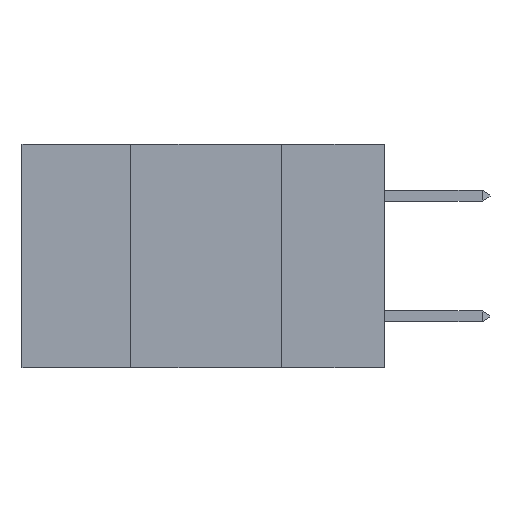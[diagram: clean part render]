
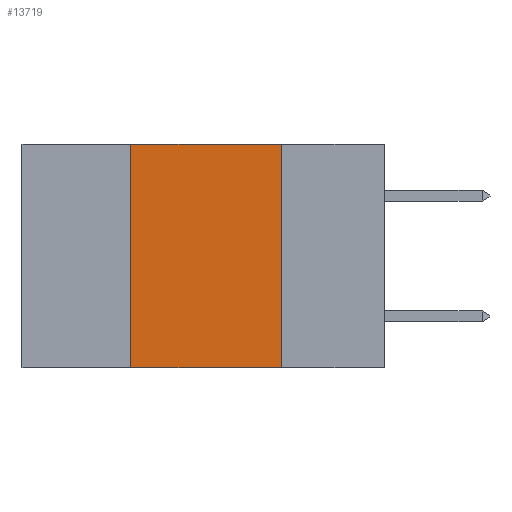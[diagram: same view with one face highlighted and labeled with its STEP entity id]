
A CAD part, left-side view. The second image highlights one B-rep face of the part: STEP entity #13719.
In plain terms, the highlighted planar face has unit normal (-1, 0, 0).
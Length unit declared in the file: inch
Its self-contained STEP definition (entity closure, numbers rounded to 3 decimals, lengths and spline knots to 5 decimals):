
#27 = CARTESIAN_POINT ( 'NONE',  ( 0., 0.6, -0.37 ) ) ;
#289 = CARTESIAN_POINT ( 'NONE',  ( 0., 0.42, -0.37 ) ) ;
#504 = ORIENTED_EDGE ( 'NONE', *, *, #11121, .F. ) ;
#980 = ORIENTED_EDGE ( 'NONE', *, *, #2295, .F. ) ;
#1001 = DIRECTION ( 'NONE',  ( 0., 0., -1. ) ) ;
#1009 = ORIENTED_EDGE ( 'NONE', *, *, #1253, .T. ) ;
#1253 = EDGE_CURVE ( 'NONE', #7658, #1440, #7962, .T. ) ;
#1312 = EDGE_LOOP ( 'NONE', ( #10034, #504, #980, #1009 ) ) ;
#1317 = VERTEX_POINT ( 'NONE', #10123 ) ;
#1440 = VERTEX_POINT ( 'NONE', #9318 ) ;
#2071 = CARTESIAN_POINT ( 'NONE',  ( 0., 0.17, 0. ) ) ;
#2295 = EDGE_CURVE ( 'NONE', #7658, #1317, #9080, .T. ) ;
#2591 = VECTOR ( 'NONE', #1001, 39.37008 ) ;
#2824 = CARTESIAN_POINT ( 'NONE',  ( 0., 0.6, 0. ) ) ;
#3166 = LINE ( 'NONE', #2071, #2591 ) ;
#3361 = AXIS2_PLACEMENT_3D ( 'NONE', #4995, #5980, #13725 ) ;
#4399 = DIRECTION ( 'NONE',  ( 0., -1., 0. ) ) ;
#4995 = CARTESIAN_POINT ( 'NONE',  ( 0., 0.6, 0. ) ) ;
#5980 = DIRECTION ( 'NONE',  ( 1., 0., 0. ) ) ;
#6031 = VECTOR ( 'NONE', #10352, 39.37008 ) ;
#6054 = FACE_OUTER_BOUND ( 'NONE', #1312, .T. ) ;
#7658 = VERTEX_POINT ( 'NONE', #289 ) ;
#7962 = LINE ( 'NONE', #27, #9209 ) ;
#8652 = CARTESIAN_POINT ( 'NONE',  ( 0., 0.17, 0. ) ) ;
#8832 = EDGE_CURVE ( 'NONE', #11739, #1440, #3166, .T. ) ;
#9080 = LINE ( 'NONE', #11172, #12213 ) ;
#9209 = VECTOR ( 'NONE', #4399, 39.37008 ) ;
#9318 = CARTESIAN_POINT ( 'NONE',  ( 0., 0.17, -0.37 ) ) ;
#10034 = ORIENTED_EDGE ( 'NONE', *, *, #8832, .F. ) ;
#10123 = CARTESIAN_POINT ( 'NONE',  ( 0., 0.42, 0. ) ) ;
#10236 = DIRECTION ( 'NONE',  ( 0., 0., 1. ) ) ;
#10352 = DIRECTION ( 'NONE',  ( 0., -1., 0. ) ) ;
#11121 = EDGE_CURVE ( 'NONE', #1317, #11739, #12621, .T. ) ;
#11172 = CARTESIAN_POINT ( 'NONE',  ( 0., 0.42, 0. ) ) ;
#11578 = PLANE ( 'NONE',  #3361 ) ;
#11739 = VERTEX_POINT ( 'NONE', #8652 ) ;
#12213 = VECTOR ( 'NONE', #10236, 39.37008 ) ;
#12621 = LINE ( 'NONE', #2824, #6031 ) ;
#13719 = ADVANCED_FACE ( 'NONE', ( #6054 ), #11578, .F. ) ;
#13725 = DIRECTION ( 'NONE',  ( 0., 0., -1. ) ) ;
